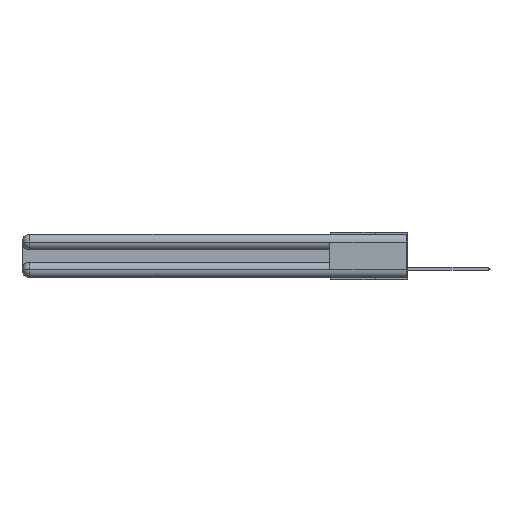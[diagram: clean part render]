
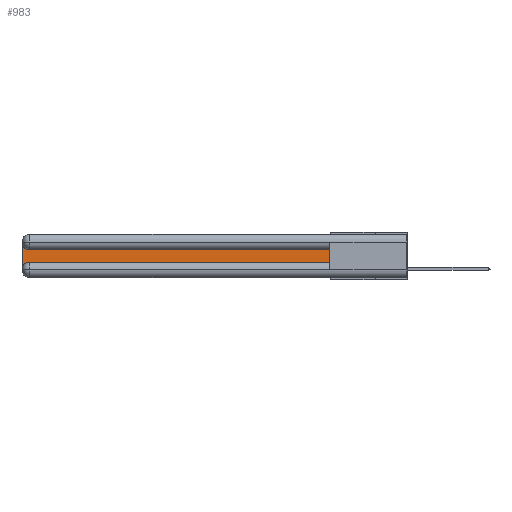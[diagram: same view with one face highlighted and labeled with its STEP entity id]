
A CAD part, left-side view. The second image highlights one B-rep face of the part: STEP entity #983.
In plain terms, the highlighted planar face has unit normal (-1, 0, 0).
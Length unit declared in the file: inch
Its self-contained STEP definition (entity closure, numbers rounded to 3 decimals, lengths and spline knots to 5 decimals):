
#373 = ORIENTED_EDGE ( 'NONE', *, *, #9166, .T. ) ;
#775 = CIRCLE ( 'NONE', #19629, 0.06 ) ;
#983 = ADVANCED_FACE ( 'NONE', ( #13411 ), #8552, .F. ) ;
#1031 = CARTESIAN_POINT ( 'NONE',  ( 0.075, 0.6, -0.1225 ) ) ;
#1104 = VERTEX_POINT ( 'NONE', #26990 ) ;
#2263 = CIRCLE ( 'NONE', #14532, 0.06 ) ;
#3127 = CARTESIAN_POINT ( 'NONE',  ( 0.075, 3., -0.2175 ) ) ;
#3693 = LINE ( 'NONE', #9964, #7566 ) ;
#3710 = CARTESIAN_POINT ( 'NONE',  ( 0.075, 2.94, -0.2775 ) ) ;
#6377 = DIRECTION ( 'NONE',  ( 1., 0., 0. ) ) ;
#7271 = VERTEX_POINT ( 'NONE', #9757 ) ;
#7566 = VECTOR ( 'NONE', #23173, 39.37008 ) ;
#7695 = CARTESIAN_POINT ( 'NONE',  ( 0.075, 2.94, -0.0625 ) ) ;
#8307 = CARTESIAN_POINT ( 'NONE',  ( 0.075, 2.94, -0.1225 ) ) ;
#8552 = PLANE ( 'NONE',  #23285 ) ;
#9166 = EDGE_CURVE ( 'NONE', #15924, #7271, #2263, .T. ) ;
#9757 = CARTESIAN_POINT ( 'NONE',  ( 0.075, 3., -0.0625 ) ) ;
#9943 = DIRECTION ( 'NONE',  ( 1., 0., 0. ) ) ;
#9964 = CARTESIAN_POINT ( 'NONE',  ( 0.075, 0.6, -0.2175 ) ) ;
#10085 = EDGE_CURVE ( 'NONE', #1104, #15924, #18146, .T. ) ;
#10276 = LINE ( 'NONE', #27706, #21479 ) ;
#10296 = DIRECTION ( 'NONE',  ( 1., 0., 0. ) ) ;
#11365 = EDGE_CURVE ( 'NONE', #25664, #1104, #3693, .T. ) ;
#12348 = DIRECTION ( 'NONE',  ( 0., 0., -1. ) ) ;
#13292 = EDGE_CURVE ( 'NONE', #24006, #18255, #775, .T. ) ;
#13411 = FACE_OUTER_BOUND ( 'NONE', #18088, .T. ) ;
#13862 = ORIENTED_EDGE ( 'NONE', *, *, #10085, .T. ) ;
#14353 = CARTESIAN_POINT ( 'NONE',  ( 0.075, 2.94, -0.2175 ) ) ;
#14464 = DIRECTION ( 'NONE',  ( 0., -1., 0. ) ) ;
#14532 = AXIS2_PLACEMENT_3D ( 'NONE', #7695, #9943, #25559 ) ;
#14602 = DIRECTION ( 'NONE',  ( 0., 0., -1. ) ) ;
#15924 = VERTEX_POINT ( 'NONE', #8307 ) ;
#16570 = DIRECTION ( 'NONE',  ( 0., 1., 0. ) ) ;
#18088 = EDGE_LOOP ( 'NONE', ( #13862, #373, #22565, #18342, #18221, #23321 ) ) ;
#18146 = LINE ( 'NONE', #1031, #21651 ) ;
#18221 = ORIENTED_EDGE ( 'NONE', *, *, #26713, .T. ) ;
#18255 = VERTEX_POINT ( 'NONE', #14353 ) ;
#18342 = ORIENTED_EDGE ( 'NONE', *, *, #13292, .T. ) ;
#18634 = CARTESIAN_POINT ( 'NONE',  ( 0.075, 0.6, -0.2175 ) ) ;
#19629 = AXIS2_PLACEMENT_3D ( 'NONE', #3710, #10296, #12348 ) ;
#21327 = VECTOR ( 'NONE', #14602, 39.37008 ) ;
#21479 = VECTOR ( 'NONE', #14464, 39.37008 ) ;
#21651 = VECTOR ( 'NONE', #16570, 39.37008 ) ;
#22565 = ORIENTED_EDGE ( 'NONE', *, *, #23499, .T. ) ;
#23173 = DIRECTION ( 'NONE',  ( 0., 0., 1. ) ) ;
#23285 = AXIS2_PLACEMENT_3D ( 'NONE', #24177, #6377, #28531 ) ;
#23321 = ORIENTED_EDGE ( 'NONE', *, *, #11365, .T. ) ;
#23499 = EDGE_CURVE ( 'NONE', #7271, #24006, #25842, .T. ) ;
#23560 = CARTESIAN_POINT ( 'NONE',  ( 0.075, 3., -0.2775 ) ) ;
#24006 = VERTEX_POINT ( 'NONE', #23560 ) ;
#24177 = CARTESIAN_POINT ( 'NONE',  ( 0.075, 3., -0.1225 ) ) ;
#25559 = DIRECTION ( 'NONE',  ( 0., 0., -1. ) ) ;
#25664 = VERTEX_POINT ( 'NONE', #18634 ) ;
#25842 = LINE ( 'NONE', #3127, #21327 ) ;
#26713 = EDGE_CURVE ( 'NONE', #18255, #25664, #10276, .T. ) ;
#26990 = CARTESIAN_POINT ( 'NONE',  ( 0.075, 0.6, -0.1225 ) ) ;
#27706 = CARTESIAN_POINT ( 'NONE',  ( 0.075, 0.6, -0.2175 ) ) ;
#28531 = DIRECTION ( 'NONE',  ( 0., 0., -1. ) ) ;
